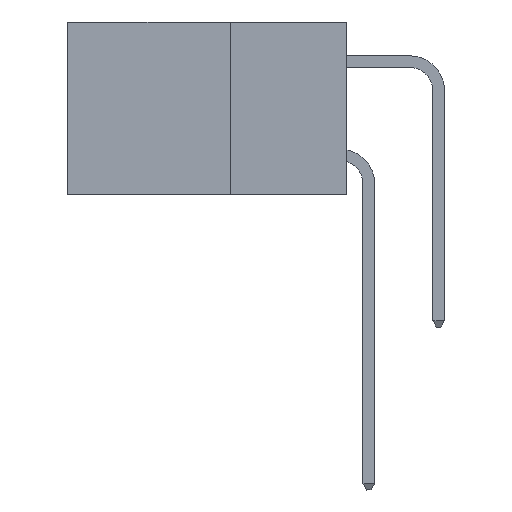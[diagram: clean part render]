
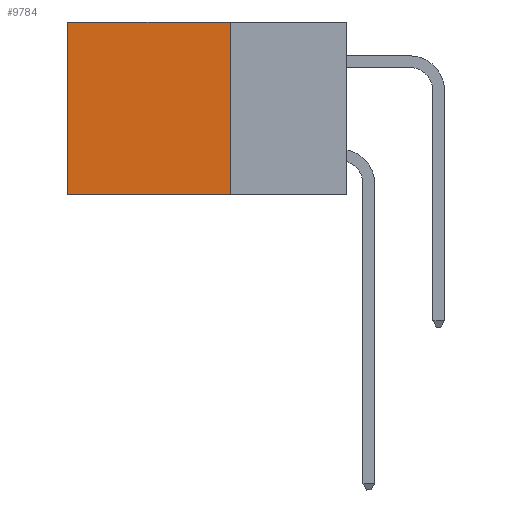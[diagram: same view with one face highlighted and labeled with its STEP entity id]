
A CAD part, left-side view. The second image highlights one B-rep face of the part: STEP entity #9784.
In plain terms, the highlighted planar face has unit normal (-1, 0, 0).
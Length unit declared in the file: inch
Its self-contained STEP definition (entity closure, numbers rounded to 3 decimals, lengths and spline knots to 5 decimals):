
#341 = VECTOR ( 'NONE', #16575, 39.37008 ) ;
#1291 = LINE ( 'NONE', #9034, #14187 ) ;
#1647 = ORIENTED_EDGE ( 'NONE', *, *, #8534, .F. ) ;
#2587 = VERTEX_POINT ( 'NONE', #5944 ) ;
#3128 = DIRECTION ( 'NONE',  ( 0., 1., 0. ) ) ;
#4185 = EDGE_LOOP ( 'NONE', ( #18123, #7531, #1647, #18392 ) ) ;
#5641 = VERTEX_POINT ( 'NONE', #19526 ) ;
#5680 = VERTEX_POINT ( 'NONE', #21178 ) ;
#5944 = CARTESIAN_POINT ( 'NONE',  ( 0.2875, 0.6, 0. ) ) ;
#6562 = VECTOR ( 'NONE', #13496, 39.37008 ) ;
#6717 = EDGE_CURVE ( 'NONE', #5641, #5680, #1291, .T. ) ;
#6773 = CARTESIAN_POINT ( 'NONE',  ( 0.2875, 0.25, 0. ) ) ;
#7531 = ORIENTED_EDGE ( 'NONE', *, *, #6717, .F. ) ;
#8534 = EDGE_CURVE ( 'NONE', #10098, #5641, #19737, .T. ) ;
#9034 = CARTESIAN_POINT ( 'NONE',  ( 0.2875, 0.25, -0.37 ) ) ;
#9438 = LINE ( 'NONE', #18205, #341 ) ;
#9784 = ADVANCED_FACE ( 'NONE', ( #19284 ), #19969, .F. ) ;
#9862 = LINE ( 'NONE', #11595, #18071 ) ;
#10098 = VERTEX_POINT ( 'NONE', #17421 ) ;
#10212 = DIRECTION ( 'NONE',  ( 1., 0., 0. ) ) ;
#11595 = CARTESIAN_POINT ( 'NONE',  ( 0.2875, 0.25, 0. ) ) ;
#11916 = CARTESIAN_POINT ( 'NONE',  ( 0.2875, 0.25, 0. ) ) ;
#13496 = DIRECTION ( 'NONE',  ( 0., 0., -1. ) ) ;
#14187 = VECTOR ( 'NONE', #20451, 39.37008 ) ;
#16290 = EDGE_CURVE ( 'NONE', #10098, #2587, #9862, .T. ) ;
#16575 = DIRECTION ( 'NONE',  ( 0., 0., -1. ) ) ;
#17421 = CARTESIAN_POINT ( 'NONE',  ( 0.2875, 0.25, 0. ) ) ;
#18071 = VECTOR ( 'NONE', #3128, 39.37008 ) ;
#18123 = ORIENTED_EDGE ( 'NONE', *, *, #20201, .T. ) ;
#18205 = CARTESIAN_POINT ( 'NONE',  ( 0.2875, 0.6, 0. ) ) ;
#18392 = ORIENTED_EDGE ( 'NONE', *, *, #16290, .T. ) ;
#19142 = AXIS2_PLACEMENT_3D ( 'NONE', #6773, #10212, #20097 ) ;
#19284 = FACE_OUTER_BOUND ( 'NONE', #4185, .T. ) ;
#19526 = CARTESIAN_POINT ( 'NONE',  ( 0.2875, 0.25, -0.37 ) ) ;
#19737 = LINE ( 'NONE', #11916, #6562 ) ;
#19969 = PLANE ( 'NONE',  #19142 ) ;
#20097 = DIRECTION ( 'NONE',  ( 0., 0., -1. ) ) ;
#20201 = EDGE_CURVE ( 'NONE', #2587, #5680, #9438, .T. ) ;
#20451 = DIRECTION ( 'NONE',  ( 0., 1., 0. ) ) ;
#21178 = CARTESIAN_POINT ( 'NONE',  ( 0.2875, 0.6, -0.37 ) ) ;
